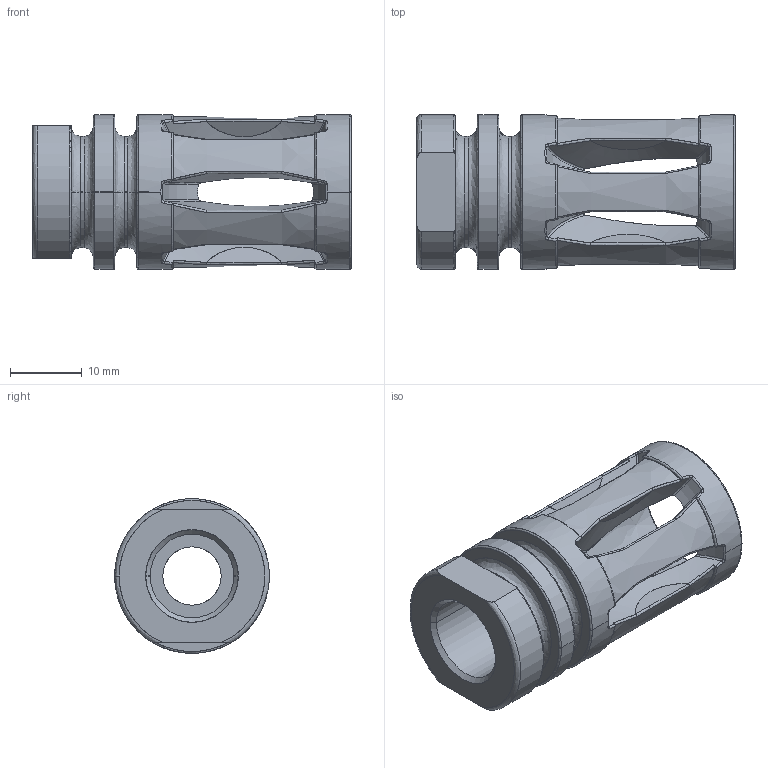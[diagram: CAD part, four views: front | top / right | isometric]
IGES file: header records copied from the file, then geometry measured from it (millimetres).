
Start section: SolidWorks IGES file using analytic representation for surfaces
Global section: file name: A-2 FH.IGS; native system: SolidWorks 2008; preprocessor: SolidWorks 2008; author: owner; date: 110731.024415; units: inch
Bounding box: 44.45 x 21.59 x 21.59 mm (x, y, z)
Surface area: 5852.7 mm2 (no closed solid volume)
Topology: 0 solids, 0 shells, 500 faces, 5451 edges, 5439 vertices
Faces by surface type: bspline 423, revolution 77
